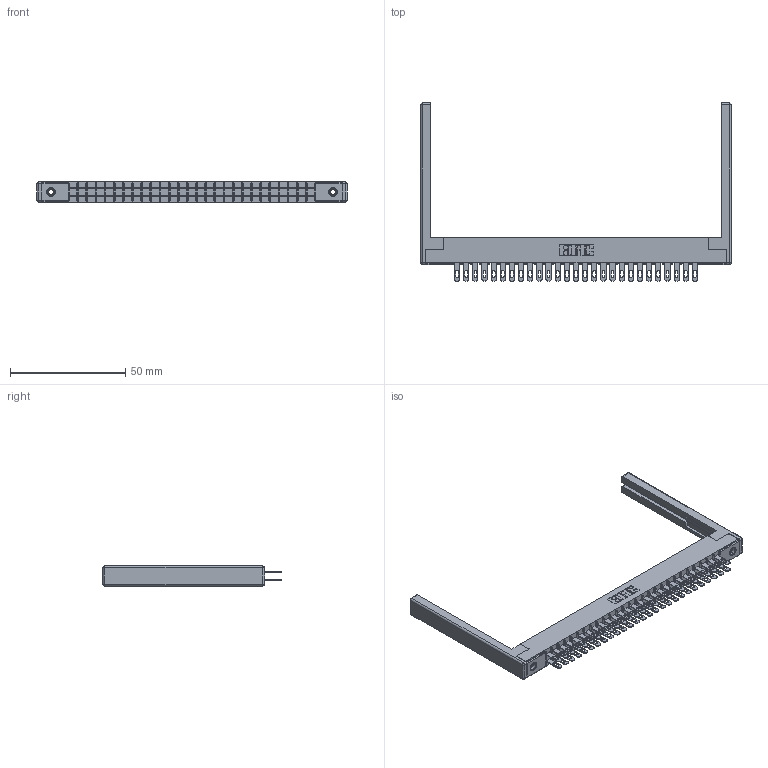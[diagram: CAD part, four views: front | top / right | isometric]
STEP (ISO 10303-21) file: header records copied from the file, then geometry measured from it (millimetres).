
FILE_DESCRIPTION (( 'STEP AP203' ), '1' );
FILE_NAME ('305-054-500-268.STEP', '2019-09-09T22:47:20', ( '' ), ( '' ), 'SwSTEP 2.0', 'SolidWorks 2016', '' );
FILE_SCHEMA (( 'CONFIG_CONTROL_DESIGN' ));
Length unit declared in the file: inch
Products named in the file (5): 305-054-500-268; 305 Part_.156 Dia; 345-250-001_345-250-001-102; 307-220-068; 305-290-001_500
Assembly tree (59 placements, depth 2):
  305-054-500-268
    305 Part_.156 Dia
    305-290-001_500  x54
    345-250-001_345-250-001-102  x2
    307-220-068  x2
Bounding box: 134.42 x 77.14 x 8.71 mm (x, y, z)
Volume: 13158.7 mm3; surface area: 21500.2 mm2
Topology: 59 solids, 59 shells, 2970 faces, 8455 edges, 5470 vertices
Faces by surface type: plane 1668, cylinder 1170, sphere 116, cone 12, torus 4
Entity records: 33841 total; most frequent: CARTESIAN_POINT 5572, ORIENTED_EDGE 5520, DIRECTION 5424, EDGE_CURVE 2760, LINE 2204, VECTOR 2204, VERTEX_POINT 1758, AXIS2_PLACEMENT_3D 1610
